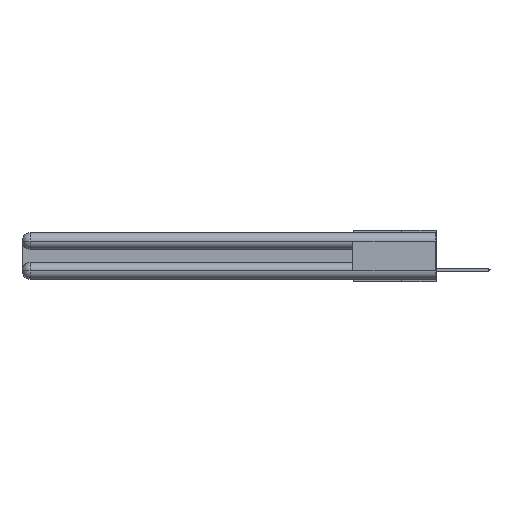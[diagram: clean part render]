
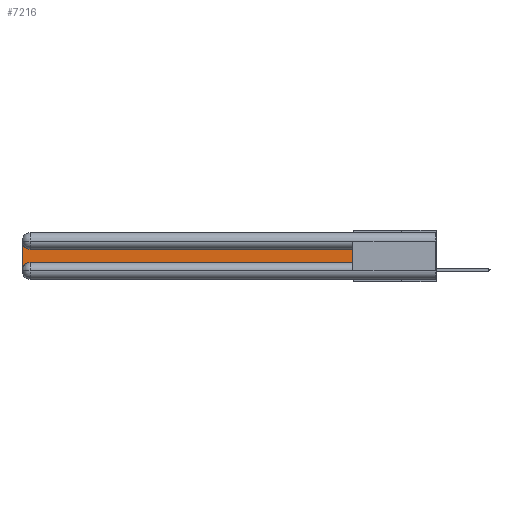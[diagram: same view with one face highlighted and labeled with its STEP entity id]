
A CAD part, left-side view. The second image highlights one B-rep face of the part: STEP entity #7216.
In plain terms, the highlighted planar face has unit normal (-1, 0, 0).
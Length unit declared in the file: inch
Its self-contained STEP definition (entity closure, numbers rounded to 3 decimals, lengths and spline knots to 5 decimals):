
#461 = CARTESIAN_POINT ( 'NONE',  ( 0.075, 3., -0.1225 ) ) ;
#2224 = LINE ( 'NONE', #18256, #21258 ) ;
#2318 = VERTEX_POINT ( 'NONE', #22471 ) ;
#2403 = VERTEX_POINT ( 'NONE', #10170 ) ;
#2555 = DIRECTION ( 'NONE',  ( 1., 0., 0. ) ) ;
#2609 = ORIENTED_EDGE ( 'NONE', *, *, #13201, .T. ) ;
#3034 = FACE_OUTER_BOUND ( 'NONE', #6719, .T. ) ;
#3423 = DIRECTION ( 'NONE',  ( 0., 1., 0. ) ) ;
#4808 = EDGE_CURVE ( 'NONE', #26045, #2318, #10549, .T. ) ;
#4921 = CARTESIAN_POINT ( 'NONE',  ( 0.075, 0.6, -0.2175 ) ) ;
#6230 = CARTESIAN_POINT ( 'NONE',  ( 0.075, 0.6, -0.1225 ) ) ;
#6683 = DIRECTION ( 'NONE',  ( 0., -1., 0. ) ) ;
#6719 = EDGE_LOOP ( 'NONE', ( #14410, #25195, #9533, #13947, #12066, #2609 ) ) ;
#6969 = CARTESIAN_POINT ( 'NONE',  ( 0.075, 2.94, -0.2175 ) ) ;
#7216 = ADVANCED_FACE ( 'NONE', ( #3034 ), #8041, .F. ) ;
#7220 = AXIS2_PLACEMENT_3D ( 'NONE', #8904, #2555, #13013 ) ;
#7717 = EDGE_CURVE ( 'NONE', #2403, #14128, #12385, .T. ) ;
#8041 = PLANE ( 'NONE',  #11845 ) ;
#8904 = CARTESIAN_POINT ( 'NONE',  ( 0.075, 2.94, -0.2775 ) ) ;
#9533 = ORIENTED_EDGE ( 'NONE', *, *, #10982, .T. ) ;
#10012 = DIRECTION ( 'NONE',  ( 0., 0., 1. ) ) ;
#10170 = CARTESIAN_POINT ( 'NONE',  ( 0.075, 2.94, -0.1225 ) ) ;
#10549 = LINE ( 'NONE', #4921, #23271 ) ;
#10982 = EDGE_CURVE ( 'NONE', #14128, #26627, #22057, .T. ) ;
#11444 = CARTESIAN_POINT ( 'NONE',  ( 0.075, 0.6, -0.1225 ) ) ;
#11845 = AXIS2_PLACEMENT_3D ( 'NONE', #461, #20980, #16737 ) ;
#12066 = ORIENTED_EDGE ( 'NONE', *, *, #4808, .T. ) ;
#12385 = CIRCLE ( 'NONE', #22966, 0.06 ) ;
#13013 = DIRECTION ( 'NONE',  ( 0., 0., -1. ) ) ;
#13201 = EDGE_CURVE ( 'NONE', #2318, #23976, #2224, .T. ) ;
#13809 = DIRECTION ( 'NONE',  ( 1., 0., 0. ) ) ;
#13947 = ORIENTED_EDGE ( 'NONE', *, *, #20879, .T. ) ;
#14128 = VERTEX_POINT ( 'NONE', #23793 ) ;
#14410 = ORIENTED_EDGE ( 'NONE', *, *, #18607, .T. ) ;
#16480 = VECTOR ( 'NONE', #3423, 39.37008 ) ;
#16737 = DIRECTION ( 'NONE',  ( 0., 0., -1. ) ) ;
#17964 = CARTESIAN_POINT ( 'NONE',  ( 0.075, 2.94, -0.0625 ) ) ;
#18256 = CARTESIAN_POINT ( 'NONE',  ( 0.075, 0.6, -0.2175 ) ) ;
#18607 = EDGE_CURVE ( 'NONE', #23976, #2403, #23871, .T. ) ;
#20127 = DIRECTION ( 'NONE',  ( 0., 0., -1. ) ) ;
#20879 = EDGE_CURVE ( 'NONE', #26627, #26045, #24992, .T. ) ;
#20980 = DIRECTION ( 'NONE',  ( 1., 0., 0. ) ) ;
#21258 = VECTOR ( 'NONE', #10012, 39.37008 ) ;
#22057 = LINE ( 'NONE', #25401, #26133 ) ;
#22471 = CARTESIAN_POINT ( 'NONE',  ( 0.075, 0.6, -0.2175 ) ) ;
#22966 = AXIS2_PLACEMENT_3D ( 'NONE', #17964, #13809, #20127 ) ;
#23271 = VECTOR ( 'NONE', #6683, 39.37008 ) ;
#23793 = CARTESIAN_POINT ( 'NONE',  ( 0.075, 3., -0.0625 ) ) ;
#23871 = LINE ( 'NONE', #11444, #16480 ) ;
#23976 = VERTEX_POINT ( 'NONE', #6230 ) ;
#24992 = CIRCLE ( 'NONE', #7220, 0.06 ) ;
#25195 = ORIENTED_EDGE ( 'NONE', *, *, #7717, .T. ) ;
#25305 = DIRECTION ( 'NONE',  ( 0., 0., -1. ) ) ;
#25401 = CARTESIAN_POINT ( 'NONE',  ( 0.075, 3., -0.2175 ) ) ;
#26045 = VERTEX_POINT ( 'NONE', #6969 ) ;
#26133 = VECTOR ( 'NONE', #25305, 39.37008 ) ;
#26627 = VERTEX_POINT ( 'NONE', #27354 ) ;
#27354 = CARTESIAN_POINT ( 'NONE',  ( 0.075, 3., -0.2775 ) ) ;
